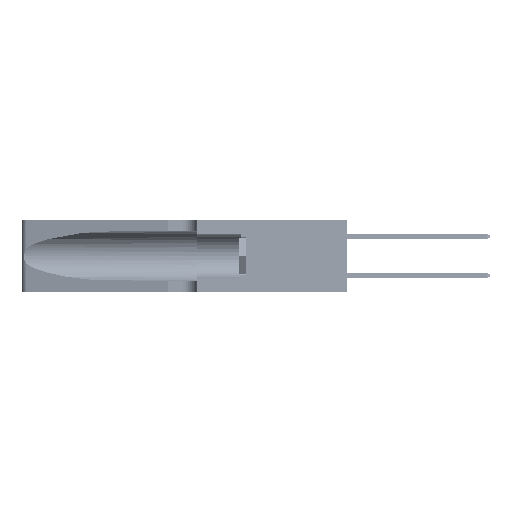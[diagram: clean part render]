
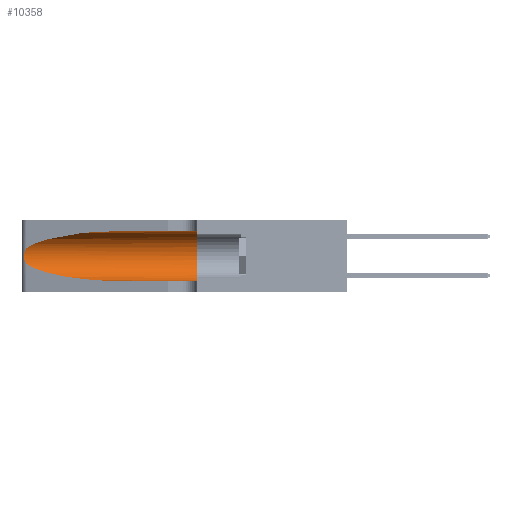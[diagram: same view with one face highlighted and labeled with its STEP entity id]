
A CAD part, left-side view. The second image highlights one B-rep face of the part: STEP entity #10358.
In plain terms, the highlighted cylindrical face has radius 3.308 mm (diameter 6.617 mm), a partial arc.
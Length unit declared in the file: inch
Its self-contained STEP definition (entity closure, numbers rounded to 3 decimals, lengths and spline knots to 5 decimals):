
#209 = DIRECTION ( 'NONE',  ( 0., -1., 0. ) ) ;
#450 = CARTESIAN_POINT ( 'NONE',  ( 0.25487, 1.22718, 0.22369 ) ) ;
#550 = B_SPLINE_CURVE_WITH_KNOTS ( 'NONE', 3,
 ( #37206, #14541, #22201, #47951, #3262, #29394, #36896, #36736, #14844, #29889, #7491, #15006, #44388, #7337 ),
 .UNSPECIFIED., .F., .F.,
 ( 4, 2, 2, 2, 2, 2, 4 ),
 ( 0., 0.00027, 0.00053, 0.00107, 0.0016, 0.00187, 0.00214 ),
 .UNSPECIFIED. ) ;
#1643 = ORIENTED_EDGE ( 'NONE', *, *, #24734, .T. ) ;
#2632 = LINE ( 'NONE', #22548, #22488 ) ;
#2843 = DIRECTION ( 'NONE',  ( 0., -1., 0. ) ) ;
#3262 = CARTESIAN_POINT ( 'NONE',  ( 0.25854, 1.2359, 0.20912 ) ) ;
#3966 = ORIENTED_EDGE ( 'NONE', *, *, #5950, .F. ) ;
#4029 = CARTESIAN_POINT ( 'NONE',  ( 0.1305, 0.72297, 0.05475 ) ) ;
#5659 = DIRECTION ( 'NONE',  ( 0., 0., -1. ) ) ;
#5771 = CARTESIAN_POINT ( 'NONE',  ( 0.18966, 0.96281, 0.31525 ) ) ;
#5950 = EDGE_CURVE ( 'NONE', #30857, #40498, #2632, .T. ) ;
#7337 = CARTESIAN_POINT ( 'NONE',  ( 0.25487, 1.22718, 0.14631 ) ) ;
#7491 = CARTESIAN_POINT ( 'NONE',  ( 0.25789, 1.23486, 0.15765 ) ) ;
#9105 = DIRECTION ( 'NONE',  ( 0., -1., 0. ) ) ;
#10358 = ADVANCED_FACE ( 'NONE', ( #41327 ), #18134, .F. ) ;
#11263 = AXIS2_PLACEMENT_3D ( 'NONE', #38489, #9105, #5659 ) ;
#14496 = DIRECTION ( 'NONE',  ( 0., 0., 1. ) ) ;
#14541 = CARTESIAN_POINT ( 'NONE',  ( 0.25555, 1.22994, 0.2215 ) ) ;
#14844 = CARTESIAN_POINT ( 'NONE',  ( 0.26017, 1.23833, 0.17102 ) ) ;
#15006 = CARTESIAN_POINT ( 'NONE',  ( 0.25639, 1.23186, 0.15144 ) ) ;
#18134 = CYLINDRICAL_SURFACE ( 'NONE', #11263, 0.13025 ) ;
#18521 = CARTESIAN_POINT ( 'NONE',  ( 0.1305, 0.35, 0.05475 ) ) ;
#19369 =( BOUNDED_CURVE ( )  B_SPLINE_CURVE ( 3, ( #45308, #33571, #22967, #4029 ),
 .UNSPECIFIED., .F., .F. ) 
 B_SPLINE_CURVE_WITH_KNOTS ( ( 4, 4 ),
 ( 3.44316, 4.71239 ),
 .UNSPECIFIED. ) 
 CURVE ( )  GEOMETRIC_REPRESENTATION_ITEM ( )  RATIONAL_B_SPLINE_CURVE ( ( 1., 0.87, 0.87, 1. ) ) 
 REPRESENTATION_ITEM ( '' )  );
#21619 = CARTESIAN_POINT ( 'NONE',  ( 0.1305, 1.61858, 0.05475 ) ) ;
#22201 = CARTESIAN_POINT ( 'NONE',  ( 0.25639, 1.23184, 0.21858 ) ) ;
#22488 = VECTOR ( 'NONE', #209, 39.37008 ) ;
#22548 = CARTESIAN_POINT ( 'NONE',  ( 0.1305, 1.61858, 0.31525 ) ) ;
#22905 = CARTESIAN_POINT ( 'NONE',  ( 0.1305, 0.35, 0.31525 ) ) ;
#22967 = CARTESIAN_POINT ( 'NONE',  ( 0.18966, 0.96281, 0.05475 ) ) ;
#23864 =( BOUNDED_CURVE ( )  B_SPLINE_CURVE ( 3, ( #24739, #5771, #39717, #24436 ),
 .UNSPECIFIED., .F., .F. ) 
 B_SPLINE_CURVE_WITH_KNOTS ( ( 4, 4 ),
 ( 1.5708, 2.84003 ),
 .UNSPECIFIED. ) 
 CURVE ( )  GEOMETRIC_REPRESENTATION_ITEM ( )  RATIONAL_B_SPLINE_CURVE ( ( 1., 0.87, 0.87, 1. ) ) 
 REPRESENTATION_ITEM ( '' )  );
#24436 = CARTESIAN_POINT ( 'NONE',  ( 0.25487, 1.22718, 0.22369 ) ) ;
#24734 = EDGE_CURVE ( 'NONE', #24960, #33987, #19369, .T. ) ;
#24739 = CARTESIAN_POINT ( 'NONE',  ( 0.1305, 0.72297, 0.31525 ) ) ;
#24960 = VERTEX_POINT ( 'NONE', #35186 ) ;
#25903 = DIRECTION ( 'NONE',  ( 0., 1., 0. ) ) ;
#28000 = VECTOR ( 'NONE', #2843, 39.37008 ) ;
#28873 = EDGE_CURVE ( 'NONE', #42254, #24960, #550, .T. ) ;
#29394 = CARTESIAN_POINT ( 'NONE',  ( 0.26018, 1.23835, 0.19895 ) ) ;
#29889 = CARTESIAN_POINT ( 'NONE',  ( 0.25856, 1.23593, 0.16098 ) ) ;
#30358 = LINE ( 'NONE', #21619, #28000 ) ;
#30455 = CIRCLE ( 'NONE', #40736, 0.13025 ) ;
#30857 = VERTEX_POINT ( 'NONE', #34120 ) ;
#32552 = ORIENTED_EDGE ( 'NONE', *, *, #36148, .T. ) ;
#33571 = CARTESIAN_POINT ( 'NONE',  ( 0.2373, 1.15595, 0.08982 ) ) ;
#33692 = ORIENTED_EDGE ( 'NONE', *, *, #42127, .F. ) ;
#33987 = VERTEX_POINT ( 'NONE', #37816 ) ;
#34120 = CARTESIAN_POINT ( 'NONE',  ( 0.1305, 0.72297, 0.31525 ) ) ;
#35186 = CARTESIAN_POINT ( 'NONE',  ( 0.25487, 1.22718, 0.14631 ) ) ;
#35854 = EDGE_LOOP ( 'NONE', ( #46485, #38376, #1643, #32552, #33692, #3966 ) ) ;
#36148 = EDGE_CURVE ( 'NONE', #33987, #36342, #30358, .T. ) ;
#36342 = VERTEX_POINT ( 'NONE', #18521 ) ;
#36736 = CARTESIAN_POINT ( 'NONE',  ( 0.26075, 1.23896, 0.178 ) ) ;
#36848 = CARTESIAN_POINT ( 'NONE',  ( 0.1305, 0.35, 0.185 ) ) ;
#36896 = CARTESIAN_POINT ( 'NONE',  ( 0.26075, 1.23896, 0.19203 ) ) ;
#37206 = CARTESIAN_POINT ( 'NONE',  ( 0.25487, 1.22718, 0.22369 ) ) ;
#37816 = CARTESIAN_POINT ( 'NONE',  ( 0.1305, 0.72297, 0.05475 ) ) ;
#38376 = ORIENTED_EDGE ( 'NONE', *, *, #28873, .T. ) ;
#38489 = CARTESIAN_POINT ( 'NONE',  ( 0.1305, 1.61858, 0.185 ) ) ;
#39717 = CARTESIAN_POINT ( 'NONE',  ( 0.2373, 1.15595, 0.28018 ) ) ;
#40498 = VERTEX_POINT ( 'NONE', #22905 ) ;
#40736 = AXIS2_PLACEMENT_3D ( 'NONE', #36848, #25903, #14496 ) ;
#41327 = FACE_OUTER_BOUND ( 'NONE', #35854, .T. ) ;
#42127 = EDGE_CURVE ( 'NONE', #40498, #36342, #30455, .T. ) ;
#42254 = VERTEX_POINT ( 'NONE', #450 ) ;
#44388 = CARTESIAN_POINT ( 'NONE',  ( 0.25555, 1.22993, 0.14849 ) ) ;
#44535 = EDGE_CURVE ( 'NONE', #30857, #42254, #23864, .T. ) ;
#45308 = CARTESIAN_POINT ( 'NONE',  ( 0.25487, 1.22718, 0.14631 ) ) ;
#46485 = ORIENTED_EDGE ( 'NONE', *, *, #44535, .T. ) ;
#47951 = CARTESIAN_POINT ( 'NONE',  ( 0.25787, 1.23484, 0.2124 ) ) ;
